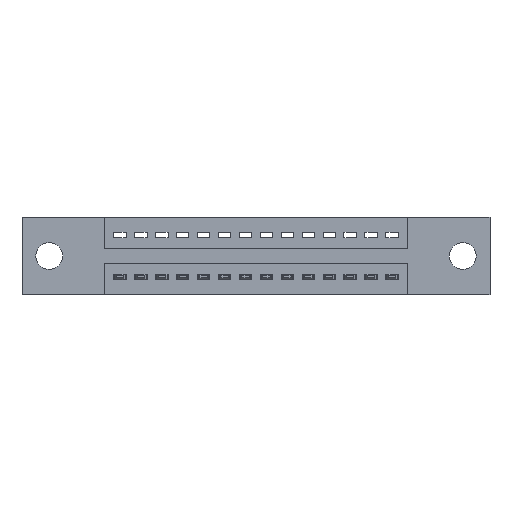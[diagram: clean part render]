
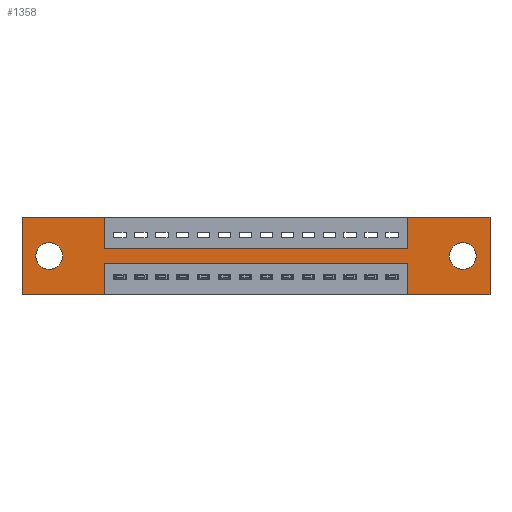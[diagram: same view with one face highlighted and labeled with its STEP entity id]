
A CAD part, front view. The second image highlights one B-rep face of the part: STEP entity #1358.
In plain terms, the highlighted planar face has unit normal (0, -1, 0).
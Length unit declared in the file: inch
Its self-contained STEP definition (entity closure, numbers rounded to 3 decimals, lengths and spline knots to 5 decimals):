
#85 = DIRECTION ( 'NONE',  ( -1., 0., 0. ) ) ;
#154 = VECTOR ( 'NONE', #5535, 39.37008 ) ;
#246 = DIRECTION ( 'NONE',  ( 0., -1., 0. ) ) ;
#383 = LINE ( 'NONE', #2858, #8340 ) ;
#473 = LINE ( 'NONE', #9409, #7251 ) ;
#504 = LINE ( 'NONE', #5343, #5568 ) ;
#886 = CARTESIAN_POINT ( 'NONE',  ( 0., 0., 0. ) ) ;
#1013 = ORIENTED_EDGE ( 'NONE', *, *, #9756, .T. ) ;
#1346 = VERTEX_POINT ( 'NONE', #9866 ) ;
#1358 = ADVANCED_FACE ( 'NONE', ( #11862, #4377, #11509 ), #3502, .T. ) ;
#1428 = VECTOR ( 'NONE', #3116, 39.37008 ) ;
#1452 = EDGE_CURVE ( 'NONE', #1537, #12296, #5697, .T. ) ;
#1537 = VERTEX_POINT ( 'NONE', #6177 ) ;
#1547 = AXIS2_PLACEMENT_3D ( 'NONE', #13452, #6892, #7982 ) ;
#1586 = EDGE_CURVE ( 'NONE', #4076, #5111, #7886, .T. ) ;
#1673 = CARTESIAN_POINT ( 'NONE',  ( 2.105, 0., -0.185 ) ) ;
#1928 = VERTEX_POINT ( 'NONE', #3159 ) ;
#1933 = LINE ( 'NONE', #6428, #9872 ) ;
#1958 = EDGE_CURVE ( 'NONE', #8129, #12659, #13055, .T. ) ;
#2193 = EDGE_CURVE ( 'NONE', #12296, #8704, #6199, .T. ) ;
#2280 = VECTOR ( 'NONE', #10360, 39.37008 ) ;
#2365 = VECTOR ( 'NONE', #8271, 39.37008 ) ;
#2387 = EDGE_CURVE ( 'NONE', #3467, #4088, #10260, .T. ) ;
#2532 = ORIENTED_EDGE ( 'NONE', *, *, #5610, .F. ) ;
#2575 = DIRECTION ( 'NONE',  ( 0., 1., 0. ) ) ;
#2595 = DIRECTION ( 'NONE',  ( -1., 0., 0. ) ) ;
#2741 = CARTESIAN_POINT ( 'NONE',  ( 0., 0., -0.37 ) ) ;
#2801 = ORIENTED_EDGE ( 'NONE', *, *, #13692, .F. ) ;
#2858 = CARTESIAN_POINT ( 'NONE',  ( 1.8425, 0., -0.37 ) ) ;
#3060 = CARTESIAN_POINT ( 'NONE',  ( 0., 0., 0. ) ) ;
#3116 = DIRECTION ( 'NONE',  ( 0., 0., 1. ) ) ;
#3159 = CARTESIAN_POINT ( 'NONE',  ( 0.3925, 0., 0. ) ) ;
#3236 = CARTESIAN_POINT ( 'NONE',  ( 0.13, 0., -0.249 ) ) ;
#3325 = LINE ( 'NONE', #10744, #2280 ) ;
#3421 = ORIENTED_EDGE ( 'NONE', *, *, #12332, .T. ) ;
#3467 = VERTEX_POINT ( 'NONE', #4682 ) ;
#3502 = PLANE ( 'NONE',  #14071 ) ;
#3793 = DIRECTION ( 'NONE',  ( 0., 0., -1. ) ) ;
#4076 = VERTEX_POINT ( 'NONE', #3236 ) ;
#4088 = VERTEX_POINT ( 'NONE', #10751 ) ;
#4206 = AXIS2_PLACEMENT_3D ( 'NONE', #1673, #4981, #13669 ) ;
#4272 = EDGE_CURVE ( 'NONE', #5449, #1537, #1933, .T. ) ;
#4354 = VECTOR ( 'NONE', #2595, 39.37008 ) ;
#4377 = FACE_BOUND ( 'NONE', #7565, .T. ) ;
#4591 = CARTESIAN_POINT ( 'NONE',  ( 1.8425, 0., -0.22 ) ) ;
#4682 = CARTESIAN_POINT ( 'NONE',  ( 2.105, 0., -0.121 ) ) ;
#4774 = CARTESIAN_POINT ( 'NONE',  ( 1.8425, 0., -0.37 ) ) ;
#4981 = DIRECTION ( 'NONE',  ( 0., 1., 0. ) ) ;
#5111 = VERTEX_POINT ( 'NONE', #12029 ) ;
#5260 = LINE ( 'NONE', #12799, #2365 ) ;
#5343 = CARTESIAN_POINT ( 'NONE',  ( 0.3925, 0., 0. ) ) ;
#5449 = VERTEX_POINT ( 'NONE', #11487 ) ;
#5535 = DIRECTION ( 'NONE',  ( 0., 0., -1. ) ) ;
#5568 = VECTOR ( 'NONE', #7427, 39.37008 ) ;
#5610 = EDGE_CURVE ( 'NONE', #1346, #1928, #11121, .T. ) ;
#5691 = ORIENTED_EDGE ( 'NONE', *, *, #1586, .T. ) ;
#5697 = LINE ( 'NONE', #10103, #9931 ) ;
#5872 = CIRCLE ( 'NONE', #4206, 0.064 ) ;
#6162 = ORIENTED_EDGE ( 'NONE', *, *, #2193, .F. ) ;
#6177 = CARTESIAN_POINT ( 'NONE',  ( 2.235, 0., 0. ) ) ;
#6199 = LINE ( 'NONE', #2741, #4354 ) ;
#6222 = DIRECTION ( 'NONE',  ( 0., 0., 1. ) ) ;
#6247 = CIRCLE ( 'NONE', #1547, 0.064 ) ;
#6428 = CARTESIAN_POINT ( 'NONE',  ( 0., 0., 0. ) ) ;
#6534 = CARTESIAN_POINT ( 'NONE',  ( 0., 0., -0.37 ) ) ;
#6557 = VERTEX_POINT ( 'NONE', #12712 ) ;
#6892 = DIRECTION ( 'NONE',  ( 0., 1., 0. ) ) ;
#7166 = CARTESIAN_POINT ( 'NONE',  ( 0.13, 0., -0.185 ) ) ;
#7251 = VECTOR ( 'NONE', #12740, 39.37008 ) ;
#7341 = CARTESIAN_POINT ( 'NONE',  ( 1.8425, 0., -0.15 ) ) ;
#7351 = LINE ( 'NONE', #886, #1428 ) ;
#7426 = ORIENTED_EDGE ( 'NONE', *, *, #2387, .T. ) ;
#7427 = DIRECTION ( 'NONE',  ( 0., 0., -1. ) ) ;
#7565 = EDGE_LOOP ( 'NONE', ( #1013, #5691 ) ) ;
#7677 = ORIENTED_EDGE ( 'NONE', *, *, #1958, .F. ) ;
#7726 = VECTOR ( 'NONE', #13836, 39.37008 ) ;
#7767 = ORIENTED_EDGE ( 'NONE', *, *, #1452, .F. ) ;
#7886 = CIRCLE ( 'NONE', #12020, 0.064 ) ;
#7911 = CARTESIAN_POINT ( 'NONE',  ( 0., 0., -0.37 ) ) ;
#7982 = DIRECTION ( 'NONE',  ( 0., 0., 1. ) ) ;
#8044 = ORIENTED_EDGE ( 'NONE', *, *, #14089, .F. ) ;
#8069 = VERTEX_POINT ( 'NONE', #6534 ) ;
#8096 = EDGE_LOOP ( 'NONE', ( #7426, #3421 ) ) ;
#8129 = VERTEX_POINT ( 'NONE', #4591 ) ;
#8135 = EDGE_LOOP ( 'NONE', ( #13723, #7677, #8044, #6162, #7767, #11131, #10151, #12694, #8862, #2532, #2801, #11726 ) ) ;
#8271 = DIRECTION ( 'NONE',  ( 0., 0., 1. ) ) ;
#8340 = VECTOR ( 'NONE', #13722, 39.37008 ) ;
#8704 = VERTEX_POINT ( 'NONE', #4774 ) ;
#8737 = CARTESIAN_POINT ( 'NONE',  ( 0.3925, 0., -0.22 ) ) ;
#8843 = CARTESIAN_POINT ( 'NONE',  ( 2.105, 0., -0.185 ) ) ;
#8862 = ORIENTED_EDGE ( 'NONE', *, *, #9397, .F. ) ;
#8902 = EDGE_CURVE ( 'NONE', #12659, #6557, #13116, .T. ) ;
#9141 = DIRECTION ( 'NONE',  ( 0., 0., -1. ) ) ;
#9276 = EDGE_CURVE ( 'NONE', #9369, #5449, #5260, .T. ) ;
#9369 = VERTEX_POINT ( 'NONE', #7341 ) ;
#9397 = EDGE_CURVE ( 'NONE', #1928, #12042, #504, .T. ) ;
#9409 = CARTESIAN_POINT ( 'NONE',  ( 0.3925, 0., -0.15 ) ) ;
#9756 = EDGE_CURVE ( 'NONE', #5111, #4076, #6247, .T. ) ;
#9866 = CARTESIAN_POINT ( 'NONE',  ( 0., 0., 0. ) ) ;
#9872 = VECTOR ( 'NONE', #12582, 39.37008 ) ;
#9931 = VECTOR ( 'NONE', #9141, 39.37008 ) ;
#9943 = CARTESIAN_POINT ( 'NONE',  ( 0.3925, 0., -0.37 ) ) ;
#9952 = EDGE_CURVE ( 'NONE', #12042, #9369, #473, .T. ) ;
#10103 = CARTESIAN_POINT ( 'NONE',  ( 2.235, 0., 0. ) ) ;
#10151 = ORIENTED_EDGE ( 'NONE', *, *, #9276, .F. ) ;
#10260 = CIRCLE ( 'NONE', #13150, 0.064 ) ;
#10360 = DIRECTION ( 'NONE',  ( -1., 0., 0. ) ) ;
#10744 = CARTESIAN_POINT ( 'NONE',  ( 0., 0., -0.37 ) ) ;
#10751 = CARTESIAN_POINT ( 'NONE',  ( 2.105, 0., -0.249 ) ) ;
#10905 = CARTESIAN_POINT ( 'NONE',  ( 0.3925, 0., -0.22 ) ) ;
#10951 = CARTESIAN_POINT ( 'NONE',  ( 0.3925, 0., -0.15 ) ) ;
#11121 = LINE ( 'NONE', #3060, #7726 ) ;
#11131 = ORIENTED_EDGE ( 'NONE', *, *, #4272, .F. ) ;
#11386 = CARTESIAN_POINT ( 'NONE',  ( 2.235, 0., -0.37 ) ) ;
#11487 = CARTESIAN_POINT ( 'NONE',  ( 1.8425, 0., 0. ) ) ;
#11509 = FACE_OUTER_BOUND ( 'NONE', #8135, .T. ) ;
#11726 = ORIENTED_EDGE ( 'NONE', *, *, #13042, .F. ) ;
#11862 = FACE_BOUND ( 'NONE', #8096, .T. ) ;
#12020 = AXIS2_PLACEMENT_3D ( 'NONE', #7166, #13845, #6222 ) ;
#12029 = CARTESIAN_POINT ( 'NONE',  ( 0.13, 0., -0.121 ) ) ;
#12042 = VERTEX_POINT ( 'NONE', #10951 ) ;
#12120 = DIRECTION ( 'NONE',  ( 0., 0., -1. ) ) ;
#12296 = VERTEX_POINT ( 'NONE', #11386 ) ;
#12332 = EDGE_CURVE ( 'NONE', #4088, #3467, #5872, .T. ) ;
#12582 = DIRECTION ( 'NONE',  ( 1., 0., 0. ) ) ;
#12659 = VERTEX_POINT ( 'NONE', #8737 ) ;
#12694 = ORIENTED_EDGE ( 'NONE', *, *, #9952, .F. ) ;
#12712 = CARTESIAN_POINT ( 'NONE',  ( 0.3925, 0., -0.37 ) ) ;
#12740 = DIRECTION ( 'NONE',  ( 1., 0., 0. ) ) ;
#12799 = CARTESIAN_POINT ( 'NONE',  ( 1.8425, 0., 0. ) ) ;
#13042 = EDGE_CURVE ( 'NONE', #6557, #8069, #3325, .T. ) ;
#13055 = LINE ( 'NONE', #10905, #13209 ) ;
#13116 = LINE ( 'NONE', #9943, #154 ) ;
#13150 = AXIS2_PLACEMENT_3D ( 'NONE', #8843, #2575, #12120 ) ;
#13209 = VECTOR ( 'NONE', #85, 39.37008 ) ;
#13452 = CARTESIAN_POINT ( 'NONE',  ( 0.13, 0., -0.185 ) ) ;
#13669 = DIRECTION ( 'NONE',  ( 0., 0., -1. ) ) ;
#13692 = EDGE_CURVE ( 'NONE', #8069, #1346, #7351, .T. ) ;
#13722 = DIRECTION ( 'NONE',  ( 0., 0., 1. ) ) ;
#13723 = ORIENTED_EDGE ( 'NONE', *, *, #8902, .F. ) ;
#13836 = DIRECTION ( 'NONE',  ( 1., 0., 0. ) ) ;
#13845 = DIRECTION ( 'NONE',  ( 0., 1., 0. ) ) ;
#14071 = AXIS2_PLACEMENT_3D ( 'NONE', #7911, #246, #3793 ) ;
#14089 = EDGE_CURVE ( 'NONE', #8704, #8129, #383, .T. ) ;
